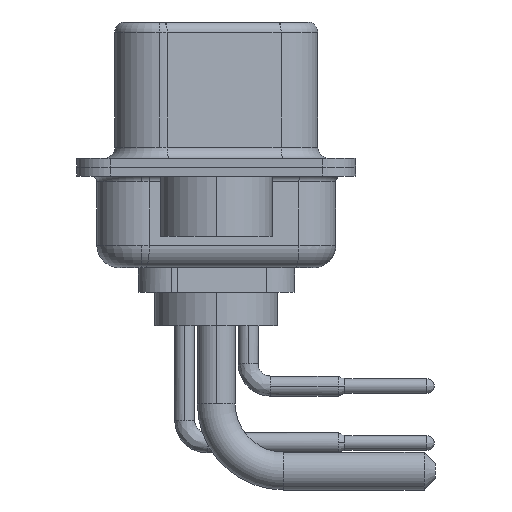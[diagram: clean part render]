
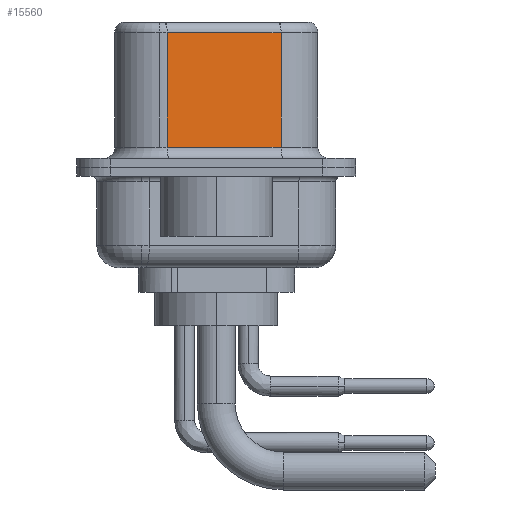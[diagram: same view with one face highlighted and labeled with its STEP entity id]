
A CAD part, left-side view. The second image highlights one B-rep face of the part: STEP entity #15560.
In plain terms, the highlighted planar face has unit normal (-0.985, -0.174, 0).
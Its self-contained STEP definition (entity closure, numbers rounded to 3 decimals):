
#513 = CARTESIAN_POINT ( 'NONE',  ( 3.68, 2.203, 0.9 ) ) ;
#556 = ORIENTED_EDGE ( 'NONE', *, *, #7345, .T. ) ;
#846 = CARTESIAN_POINT ( 'NONE',  ( 4.58, -2.897, 0.9 ) ) ;
#1247 = DIRECTION ( 'NONE',  ( 0.174, -0.985, 0. ) ) ;
#2561 = CARTESIAN_POINT ( 'NONE',  ( 4.58, -2.897, 6.52 ) ) ;
#2857 = LINE ( 'NONE', #16243, #5100 ) ;
#3335 = DIRECTION ( 'NONE',  ( -0.174, 0.985, 0. ) ) ;
#3588 = PLANE ( 'NONE',  #17355 ) ;
#4961 = ORIENTED_EDGE ( 'NONE', *, *, #18792, .T. ) ;
#5100 = VECTOR ( 'NONE', #1247, 1000. ) ;
#6234 = DIRECTION ( 'NONE',  ( -0.174, 0.985, 0. ) ) ;
#7345 = EDGE_CURVE ( 'NONE', #23187, #15305, #17396, .T. ) ;
#8086 = CARTESIAN_POINT ( 'NONE',  ( 4.58, -2.897, 6.02 ) ) ;
#8146 = DIRECTION ( 'NONE',  ( 0., 0., -1. ) ) ;
#8476 = VECTOR ( 'NONE', #8146, 1000. ) ;
#8786 = VECTOR ( 'NONE', #6234, 1000. ) ;
#9921 = CARTESIAN_POINT ( 'NONE',  ( 4.58, -2.897, 6.02 ) ) ;
#11215 = EDGE_CURVE ( 'NONE', #19544, #23188, #15824, .T. ) ;
#12285 = VECTOR ( 'NONE', #21002, 1000. ) ;
#12516 = ORIENTED_EDGE ( 'NONE', *, *, #19797, .T. ) ;
#12992 = FACE_OUTER_BOUND ( 'NONE', #18516, .T. ) ;
#13337 = ORIENTED_EDGE ( 'NONE', *, *, #11215, .F. ) ;
#15305 = VERTEX_POINT ( 'NONE', #513 ) ;
#15560 = ADVANCED_FACE ( 'NONE', ( #12992 ), #3588, .F. ) ;
#15824 = LINE ( 'NONE', #2561, #8476 ) ;
#16235 = CARTESIAN_POINT ( 'NONE',  ( 4.58, -2.897, 6.52 ) ) ;
#16243 = CARTESIAN_POINT ( 'NONE',  ( 4.58, -2.897, 0.9 ) ) ;
#17355 = AXIS2_PLACEMENT_3D ( 'NONE', #16235, #20606, #3335 ) ;
#17396 = LINE ( 'NONE', #20888, #12285 ) ;
#18516 = EDGE_LOOP ( 'NONE', ( #13337, #12516, #556, #4961 ) ) ;
#18792 = EDGE_CURVE ( 'NONE', #15305, #23188, #2857, .T. ) ;
#19335 = CARTESIAN_POINT ( 'NONE',  ( 3.68, 2.203, 6.02 ) ) ;
#19544 = VERTEX_POINT ( 'NONE', #9921 ) ;
#19797 = EDGE_CURVE ( 'NONE', #19544, #23187, #21627, .T. ) ;
#20606 = DIRECTION ( 'NONE',  ( 0.985, 0.174, 0. ) ) ;
#20888 = CARTESIAN_POINT ( 'NONE',  ( 3.68, 2.203, 6.52 ) ) ;
#21002 = DIRECTION ( 'NONE',  ( 0., 0., -1. ) ) ;
#21627 = LINE ( 'NONE', #8086, #8786 ) ;
#23187 = VERTEX_POINT ( 'NONE', #19335 ) ;
#23188 = VERTEX_POINT ( 'NONE', #846 ) ;
